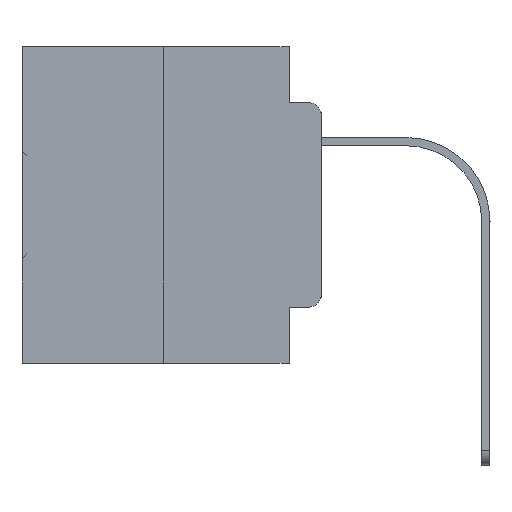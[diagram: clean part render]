
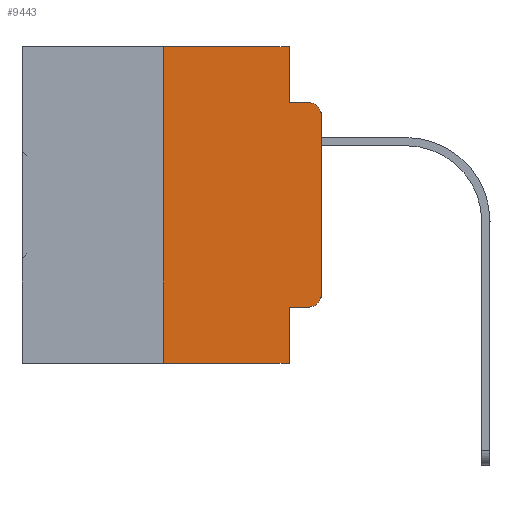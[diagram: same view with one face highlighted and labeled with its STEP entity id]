
A CAD part, left-side view. The second image highlights one B-rep face of the part: STEP entity #9443.
In plain terms, the highlighted planar face has unit normal (-1, 0, 0).
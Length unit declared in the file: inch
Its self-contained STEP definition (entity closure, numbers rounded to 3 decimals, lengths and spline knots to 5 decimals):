
#269 = LINE ( 'NONE', #32683, #1698 ) ;
#427 = EDGE_CURVE ( 'NONE', #27043, #3640, #17845, .T. ) ;
#476 = VERTEX_POINT ( 'NONE', #16744 ) ;
#768 = CIRCLE ( 'NONE', #5060, 0.02 ) ;
#1111 = EDGE_CURVE ( 'NONE', #13142, #27200, #32311, .T. ) ;
#1492 = EDGE_LOOP ( 'NONE', ( #7651, #1979, #15403, #25693, #26814, #10476, #11845, #18340, #23278, #21545 ) ) ;
#1698 = VECTOR ( 'NONE', #27556, 39.37008 ) ;
#1979 = ORIENTED_EDGE ( 'NONE', *, *, #21566, .T. ) ;
#2406 = DIRECTION ( 'NONE',  ( 0., 0., -1. ) ) ;
#2413 = VERTEX_POINT ( 'NONE', #17408 ) ;
#2541 = VECTOR ( 'NONE', #23349, 39.37008 ) ;
#2924 = CARTESIAN_POINT ( 'NONE',  ( 0., 0.051, -0.0885 ) ) ;
#3539 = LINE ( 'NONE', #4385, #23704 ) ;
#3640 = VERTEX_POINT ( 'NONE', #15581 ) ;
#4385 = CARTESIAN_POINT ( 'NONE',  ( 0., 0., 0. ) ) ;
#5060 = AXIS2_PLACEMENT_3D ( 'NONE', #27011, #29504, #18863 ) ;
#5761 = DIRECTION ( 'NONE',  ( 0., 0., -1. ) ) ;
#6065 = VECTOR ( 'NONE', #2406, 39.37008 ) ;
#7581 = LINE ( 'NONE', #15557, #6065 ) ;
#7651 = ORIENTED_EDGE ( 'NONE', *, *, #18163, .T. ) ;
#7759 = AXIS2_PLACEMENT_3D ( 'NONE', #10180, #11100, #21222 ) ;
#9258 = CARTESIAN_POINT ( 'NONE',  ( 0., 0.25, 0. ) ) ;
#9443 = ADVANCED_FACE ( 'NONE', ( #23850 ), #31007, .F. ) ;
#9560 = CARTESIAN_POINT ( 'NONE',  ( 0., 0.473, -0.5 ) ) ;
#9827 = CARTESIAN_POINT ( 'NONE',  ( 0., 0.051, 0. ) ) ;
#10180 = CARTESIAN_POINT ( 'NONE',  ( 0., 0.02, -0.3915 ) ) ;
#10476 = ORIENTED_EDGE ( 'NONE', *, *, #29791, .F. ) ;
#10751 = DIRECTION ( 'NONE',  ( 1., 0., 0. ) ) ;
#11053 = VERTEX_POINT ( 'NONE', #17338 ) ;
#11100 = DIRECTION ( 'NONE',  ( -1., 0., 0. ) ) ;
#11113 = VERTEX_POINT ( 'NONE', #20320 ) ;
#11845 = ORIENTED_EDGE ( 'NONE', *, *, #1111, .T. ) ;
#12059 = DIRECTION ( 'NONE',  ( 0., -1., 0. ) ) ;
#13142 = VERTEX_POINT ( 'NONE', #27880 ) ;
#13966 = VERTEX_POINT ( 'NONE', #16508 ) ;
#14190 = VECTOR ( 'NONE', #12059, 39.37008 ) ;
#14349 = LINE ( 'NONE', #19484, #27029 ) ;
#15379 = CARTESIAN_POINT ( 'NONE',  ( 0., 0.051, -0.4115 ) ) ;
#15403 = ORIENTED_EDGE ( 'NONE', *, *, #18693, .F. ) ;
#15557 = CARTESIAN_POINT ( 'NONE',  ( 0., 0.051, 0. ) ) ;
#15581 = CARTESIAN_POINT ( 'NONE',  ( 0., 0., -0.3915 ) ) ;
#15734 = LINE ( 'NONE', #2924, #2541 ) ;
#16508 = CARTESIAN_POINT ( 'NONE',  ( 0., 0.051, -0.4115 ) ) ;
#16744 = CARTESIAN_POINT ( 'NONE',  ( 0., 0.051, -0.0885 ) ) ;
#17338 = CARTESIAN_POINT ( 'NONE',  ( 0., 0., -0.1085 ) ) ;
#17408 = CARTESIAN_POINT ( 'NONE',  ( 0., 0.02, -0.0885 ) ) ;
#17842 = EDGE_CURVE ( 'NONE', #13966, #27043, #30161, .T. ) ;
#17845 = CIRCLE ( 'NONE', #7759, 0.02 ) ;
#18163 = EDGE_CURVE ( 'NONE', #3640, #11053, #3539, .T. ) ;
#18340 = ORIENTED_EDGE ( 'NONE', *, *, #25672, .F. ) ;
#18693 = EDGE_CURVE ( 'NONE', #476, #2413, #15734, .T. ) ;
#18863 = DIRECTION ( 'NONE',  ( 0., 0., -1. ) ) ;
#19356 = VECTOR ( 'NONE', #29689, 39.37008 ) ;
#19484 = CARTESIAN_POINT ( 'NONE',  ( 0., 0.473, 0. ) ) ;
#19695 = DIRECTION ( 'NONE',  ( 0., -1., 0. ) ) ;
#19871 = VERTEX_POINT ( 'NONE', #9827 ) ;
#20320 = CARTESIAN_POINT ( 'NONE',  ( 0., 0.25, 0. ) ) ;
#21222 = DIRECTION ( 'NONE',  ( 0., 0., -1. ) ) ;
#21545 = ORIENTED_EDGE ( 'NONE', *, *, #427, .T. ) ;
#21566 = EDGE_CURVE ( 'NONE', #11053, #2413, #768, .T. ) ;
#21815 = CARTESIAN_POINT ( 'NONE',  ( 0., 0.02, -0.4115 ) ) ;
#21876 = LINE ( 'NONE', #9258, #19356 ) ;
#22633 = CARTESIAN_POINT ( 'NONE',  ( 0., 0.051, -0.5 ) ) ;
#23278 = ORIENTED_EDGE ( 'NONE', *, *, #17842, .T. ) ;
#23349 = DIRECTION ( 'NONE',  ( 0., -1., 0. ) ) ;
#23355 = CARTESIAN_POINT ( 'NONE',  ( 0., 0.473, 0. ) ) ;
#23704 = VECTOR ( 'NONE', #27633, 39.37008 ) ;
#23850 = FACE_OUTER_BOUND ( 'NONE', #1492, .T. ) ;
#25672 = EDGE_CURVE ( 'NONE', #13966, #27200, #269, .T. ) ;
#25693 = ORIENTED_EDGE ( 'NONE', *, *, #29861, .F. ) ;
#26814 = ORIENTED_EDGE ( 'NONE', *, *, #31956, .F. ) ;
#26958 = DIRECTION ( 'NONE',  ( 0., -1., 0. ) ) ;
#27011 = CARTESIAN_POINT ( 'NONE',  ( 0., 0.02, -0.1085 ) ) ;
#27029 = VECTOR ( 'NONE', #26958, 39.37008 ) ;
#27043 = VERTEX_POINT ( 'NONE', #21815 ) ;
#27200 = VERTEX_POINT ( 'NONE', #22633 ) ;
#27556 = DIRECTION ( 'NONE',  ( 0., 0., -1. ) ) ;
#27633 = DIRECTION ( 'NONE',  ( 0., 0., 1. ) ) ;
#27880 = CARTESIAN_POINT ( 'NONE',  ( 0., 0.25, -0.5 ) ) ;
#29504 = DIRECTION ( 'NONE',  ( -1., 0., 0. ) ) ;
#29689 = DIRECTION ( 'NONE',  ( 0., 0., 1. ) ) ;
#29791 = EDGE_CURVE ( 'NONE', #13142, #11113, #21876, .T. ) ;
#29861 = EDGE_CURVE ( 'NONE', #19871, #476, #7581, .T. ) ;
#30161 = LINE ( 'NONE', #15379, #14190 ) ;
#30641 = VECTOR ( 'NONE', #19695, 39.37008 ) ;
#31007 = PLANE ( 'NONE',  #31205 ) ;
#31205 = AXIS2_PLACEMENT_3D ( 'NONE', #23355, #10751, #5761 ) ;
#31956 = EDGE_CURVE ( 'NONE', #11113, #19871, #14349, .T. ) ;
#32311 = LINE ( 'NONE', #9560, #30641 ) ;
#32683 = CARTESIAN_POINT ( 'NONE',  ( 0., 0.051, 0. ) ) ;
